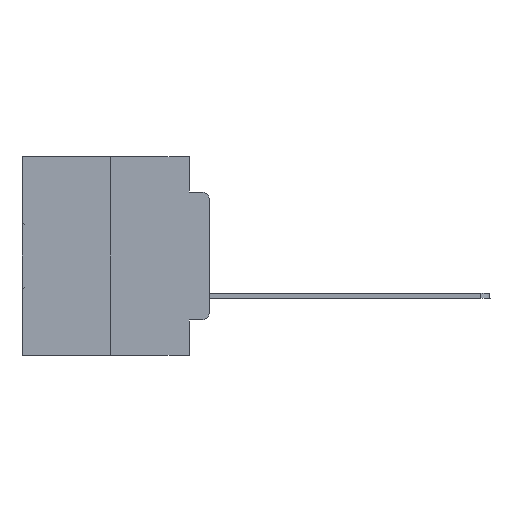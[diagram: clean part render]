
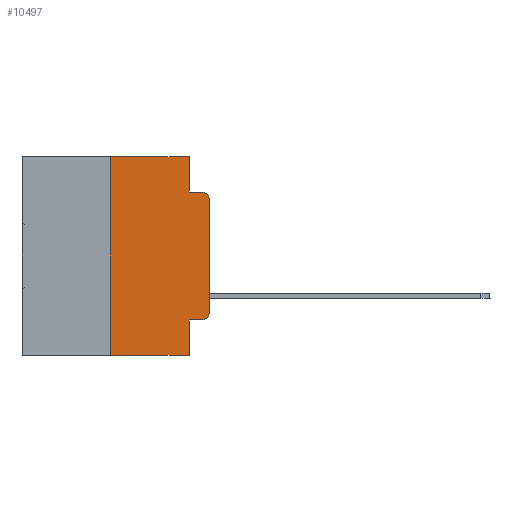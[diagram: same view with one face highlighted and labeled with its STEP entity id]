
A CAD part, left-side view. The second image highlights one B-rep face of the part: STEP entity #10497.
In plain terms, the highlighted planar face has unit normal (-1, 0, 0).
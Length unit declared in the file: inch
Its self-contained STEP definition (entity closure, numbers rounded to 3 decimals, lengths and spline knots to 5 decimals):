
#263 = EDGE_CURVE ( 'NONE', #27896, #7112, #21056, .T. ) ;
#1053 = EDGE_LOOP ( 'NONE', ( #20230, #27650, #32209, #8283, #28783, #27067, #32437, #4430, #17284, #29874 ) ) ;
#1876 = CARTESIAN_POINT ( 'NONE',  ( 0., 0.02, -0.4115 ) ) ;
#2578 = CARTESIAN_POINT ( 'NONE',  ( 0., 0.02, -0.0885 ) ) ;
#2585 = CARTESIAN_POINT ( 'NONE',  ( 0., 0.25, -0.5 ) ) ;
#3956 = DIRECTION ( 'NONE',  ( 0., 0., -1. ) ) ;
#4017 = VERTEX_POINT ( 'NONE', #30385 ) ;
#4214 = AXIS2_PLACEMENT_3D ( 'NONE', #21336, #13366, #19764 ) ;
#4430 = ORIENTED_EDGE ( 'NONE', *, *, #15021, .F. ) ;
#4455 = EDGE_CURVE ( 'NONE', #31287, #8713, #25155, .T. ) ;
#4608 = CARTESIAN_POINT ( 'NONE',  ( 0., 0.473, -0.5 ) ) ;
#4713 = DIRECTION ( 'NONE',  ( 0., -1., 0. ) ) ;
#4861 = CARTESIAN_POINT ( 'NONE',  ( 0., 0.051, 0. ) ) ;
#5042 = VECTOR ( 'NONE', #16653, 39.37008 ) ;
#5575 = EDGE_CURVE ( 'NONE', #8713, #27896, #27398, .T. ) ;
#6102 = VERTEX_POINT ( 'NONE', #2585 ) ;
#6149 = VECTOR ( 'NONE', #26786, 39.37008 ) ;
#7074 = VERTEX_POINT ( 'NONE', #13546 ) ;
#7112 = VERTEX_POINT ( 'NONE', #28771 ) ;
#7144 = DIRECTION ( 'NONE',  ( -1., 0., 0. ) ) ;
#7402 = EDGE_CURVE ( 'NONE', #6102, #4017, #15043, .T. ) ;
#8283 = ORIENTED_EDGE ( 'NONE', *, *, #13464, .F. ) ;
#8425 = EDGE_CURVE ( 'NONE', #26335, #14466, #20045, .T. ) ;
#8713 = VERTEX_POINT ( 'NONE', #1876 ) ;
#9623 = CARTESIAN_POINT ( 'NONE',  ( 0., 0.051, -0.0885 ) ) ;
#10044 = LINE ( 'NONE', #21821, #13632 ) ;
#10497 = ADVANCED_FACE ( 'NONE', ( #23030 ), #15720, .F. ) ;
#10667 = DIRECTION ( 'NONE',  ( 1., 0., 0. ) ) ;
#11350 = CARTESIAN_POINT ( 'NONE',  ( 0., 0.051, -0.4115 ) ) ;
#11364 = CIRCLE ( 'NONE', #4214, 0.02 ) ;
#12121 = LINE ( 'NONE', #29418, #6149 ) ;
#12463 = CARTESIAN_POINT ( 'NONE',  ( 0., 0., -0.3915 ) ) ;
#12896 = DIRECTION ( 'NONE',  ( 0., 0., 1. ) ) ;
#13314 = VECTOR ( 'NONE', #30962, 39.37008 ) ;
#13366 = DIRECTION ( 'NONE',  ( -1., 0., 0. ) ) ;
#13464 = EDGE_CURVE ( 'NONE', #7074, #26335, #10044, .T. ) ;
#13546 = CARTESIAN_POINT ( 'NONE',  ( 0., 0.051, 0. ) ) ;
#13632 = VECTOR ( 'NONE', #3956, 39.37008 ) ;
#13949 = CARTESIAN_POINT ( 'NONE',  ( 0., 0.25, 0. ) ) ;
#14399 = DIRECTION ( 'NONE',  ( 0., 0., -1. ) ) ;
#14466 = VERTEX_POINT ( 'NONE', #2578 ) ;
#14783 = LINE ( 'NONE', #4861, #21811 ) ;
#14896 = VERTEX_POINT ( 'NONE', #16452 ) ;
#15021 = EDGE_CURVE ( 'NONE', #31287, #4017, #14783, .T. ) ;
#15043 = LINE ( 'NONE', #4608, #30753 ) ;
#15672 = CARTESIAN_POINT ( 'NONE',  ( 0., 0.051, -0.0885 ) ) ;
#15720 = PLANE ( 'NONE',  #27883 ) ;
#16452 = CARTESIAN_POINT ( 'NONE',  ( 0., 0.25, 0. ) ) ;
#16653 = DIRECTION ( 'NONE',  ( 0., 0., 1. ) ) ;
#17284 = ORIENTED_EDGE ( 'NONE', *, *, #4455, .T. ) ;
#18345 = VECTOR ( 'NONE', #12896, 39.37008 ) ;
#19764 = DIRECTION ( 'NONE',  ( 0., 0., -1. ) ) ;
#19861 = EDGE_CURVE ( 'NONE', #6102, #14896, #20416, .T. ) ;
#19934 = CARTESIAN_POINT ( 'NONE',  ( 0., 0.051, -0.4115 ) ) ;
#20045 = LINE ( 'NONE', #15672, #13314 ) ;
#20230 = ORIENTED_EDGE ( 'NONE', *, *, #263, .T. ) ;
#20285 = CARTESIAN_POINT ( 'NONE',  ( 0., 0., 0. ) ) ;
#20416 = LINE ( 'NONE', #13949, #5042 ) ;
#20959 = DIRECTION ( 'NONE',  ( 0., 0., -1. ) ) ;
#21056 = LINE ( 'NONE', #20285, #18345 ) ;
#21336 = CARTESIAN_POINT ( 'NONE',  ( 0., 0.02, -0.1085 ) ) ;
#21811 = VECTOR ( 'NONE', #22538, 39.37008 ) ;
#21821 = CARTESIAN_POINT ( 'NONE',  ( 0., 0.051, 0. ) ) ;
#22538 = DIRECTION ( 'NONE',  ( 0., 0., -1. ) ) ;
#23030 = FACE_OUTER_BOUND ( 'NONE', #1053, .T. ) ;
#25155 = LINE ( 'NONE', #11350, #28270 ) ;
#25413 = AXIS2_PLACEMENT_3D ( 'NONE', #32258, #7144, #14399 ) ;
#26278 = EDGE_CURVE ( 'NONE', #14896, #7074, #12121, .T. ) ;
#26335 = VERTEX_POINT ( 'NONE', #9623 ) ;
#26408 = DIRECTION ( 'NONE',  ( 0., -1., 0. ) ) ;
#26786 = DIRECTION ( 'NONE',  ( 0., -1., 0. ) ) ;
#27067 = ORIENTED_EDGE ( 'NONE', *, *, #19861, .F. ) ;
#27398 = CIRCLE ( 'NONE', #25413, 0.02 ) ;
#27650 = ORIENTED_EDGE ( 'NONE', *, *, #30544, .T. ) ;
#27883 = AXIS2_PLACEMENT_3D ( 'NONE', #28591, #10667, #20959 ) ;
#27896 = VERTEX_POINT ( 'NONE', #12463 ) ;
#28270 = VECTOR ( 'NONE', #26408, 39.37008 ) ;
#28591 = CARTESIAN_POINT ( 'NONE',  ( 0., 0.473, 0. ) ) ;
#28771 = CARTESIAN_POINT ( 'NONE',  ( 0., 0., -0.1085 ) ) ;
#28783 = ORIENTED_EDGE ( 'NONE', *, *, #26278, .F. ) ;
#29418 = CARTESIAN_POINT ( 'NONE',  ( 0., 0.473, 0. ) ) ;
#29874 = ORIENTED_EDGE ( 'NONE', *, *, #5575, .T. ) ;
#30385 = CARTESIAN_POINT ( 'NONE',  ( 0., 0.051, -0.5 ) ) ;
#30544 = EDGE_CURVE ( 'NONE', #7112, #14466, #11364, .T. ) ;
#30753 = VECTOR ( 'NONE', #4713, 39.37008 ) ;
#30962 = DIRECTION ( 'NONE',  ( 0., -1., 0. ) ) ;
#31287 = VERTEX_POINT ( 'NONE', #19934 ) ;
#32209 = ORIENTED_EDGE ( 'NONE', *, *, #8425, .F. ) ;
#32258 = CARTESIAN_POINT ( 'NONE',  ( 0., 0.02, -0.3915 ) ) ;
#32437 = ORIENTED_EDGE ( 'NONE', *, *, #7402, .T. ) ;
